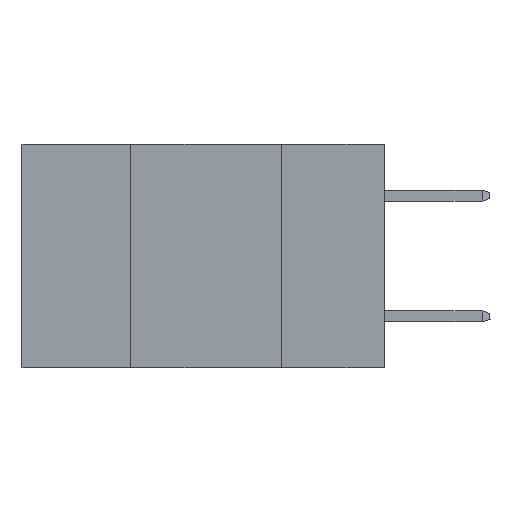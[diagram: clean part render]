
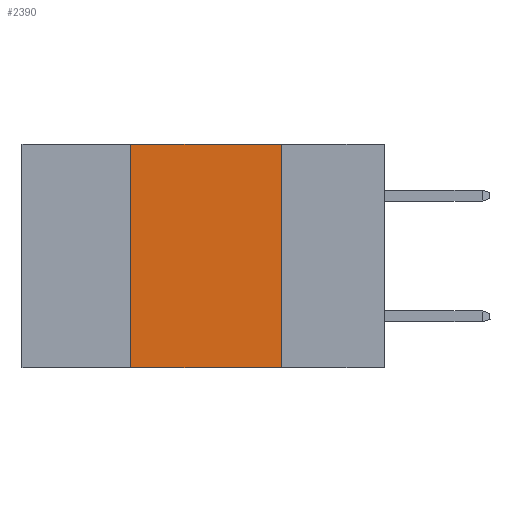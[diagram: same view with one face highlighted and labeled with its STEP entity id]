
A CAD part, left-side view. The second image highlights one B-rep face of the part: STEP entity #2390.
In plain terms, the highlighted planar face has unit normal (-1, 0, 0).
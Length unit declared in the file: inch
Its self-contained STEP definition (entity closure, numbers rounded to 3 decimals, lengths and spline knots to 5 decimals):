
#534 = VERTEX_POINT ( 'NONE', #21955 ) ;
#2260 = VECTOR ( 'NONE', #17783, 39.37008 ) ;
#2390 = ADVANCED_FACE ( 'NONE', ( #13877 ), #13784, .F. ) ;
#3038 = CARTESIAN_POINT ( 'NONE',  ( 0., 0.6, -0.37 ) ) ;
#3043 = CARTESIAN_POINT ( 'NONE',  ( 0., 0.17, -0.37 ) ) ;
#3297 = DIRECTION ( 'NONE',  ( 0., -1., 0. ) ) ;
#3323 = DIRECTION ( 'NONE',  ( 1., 0., 0. ) ) ;
#3685 = CARTESIAN_POINT ( 'NONE',  ( 0., 0.17, -0.37 ) ) ;
#3722 = EDGE_CURVE ( 'NONE', #534, #13361, #19784, .T. ) ;
#3735 = LINE ( 'NONE', #15433, #7888 ) ;
#3776 = VECTOR ( 'NONE', #16861, 39.37008 ) ;
#4118 = VERTEX_POINT ( 'NONE', #22090 ) ;
#5118 = VECTOR ( 'NONE', #10172, 39.37008 ) ;
#7602 = CARTESIAN_POINT ( 'NONE',  ( 0., 0.42, -0.37 ) ) ;
#7888 = VECTOR ( 'NONE', #3297, 39.37008 ) ;
#7961 = CARTESIAN_POINT ( 'NONE',  ( 0., 0.17, 0. ) ) ;
#8924 = EDGE_CURVE ( 'NONE', #4118, #18222, #3735, .T. ) ;
#10172 = DIRECTION ( 'NONE',  ( 0., -1., 0. ) ) ;
#13361 = VERTEX_POINT ( 'NONE', #3685 ) ;
#13521 = EDGE_CURVE ( 'NONE', #18222, #13361, #17510, .T. ) ;
#13784 = PLANE ( 'NONE',  #16515 ) ;
#13877 = FACE_OUTER_BOUND ( 'NONE', #19748, .T. ) ;
#13953 = ORIENTED_EDGE ( 'NONE', *, *, #3722, .T. ) ;
#15433 = CARTESIAN_POINT ( 'NONE',  ( 0., 0.6, 0. ) ) ;
#15457 = DIRECTION ( 'NONE',  ( 0., 0., -1. ) ) ;
#15761 = EDGE_CURVE ( 'NONE', #534, #4118, #16617, .T. ) ;
#16278 = ORIENTED_EDGE ( 'NONE', *, *, #8924, .F. ) ;
#16515 = AXIS2_PLACEMENT_3D ( 'NONE', #21656, #3323, #15457 ) ;
#16617 = LINE ( 'NONE', #7602, #2260 ) ;
#16861 = DIRECTION ( 'NONE',  ( 0., 0., -1. ) ) ;
#17510 = LINE ( 'NONE', #3043, #3776 ) ;
#17783 = DIRECTION ( 'NONE',  ( 0., 0., 1. ) ) ;
#17836 = ORIENTED_EDGE ( 'NONE', *, *, #15761, .F. ) ;
#18222 = VERTEX_POINT ( 'NONE', #7961 ) ;
#19748 = EDGE_LOOP ( 'NONE', ( #21224, #16278, #17836, #13953 ) ) ;
#19784 = LINE ( 'NONE', #3038, #5118 ) ;
#21224 = ORIENTED_EDGE ( 'NONE', *, *, #13521, .F. ) ;
#21656 = CARTESIAN_POINT ( 'NONE',  ( 0., 0.6, 0. ) ) ;
#21955 = CARTESIAN_POINT ( 'NONE',  ( 0., 0.42, -0.37 ) ) ;
#22090 = CARTESIAN_POINT ( 'NONE',  ( 0., 0.42, 0. ) ) ;
